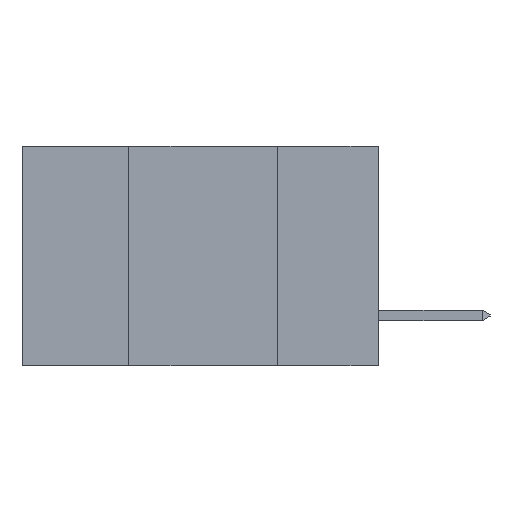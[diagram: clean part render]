
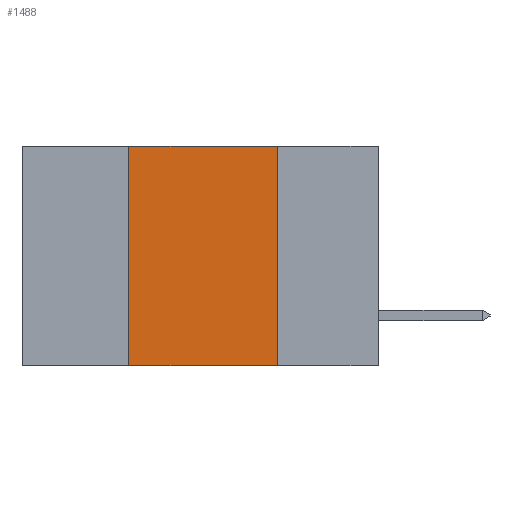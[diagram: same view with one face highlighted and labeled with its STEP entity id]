
A CAD part, left-side view. The second image highlights one B-rep face of the part: STEP entity #1488.
In plain terms, the highlighted planar face has unit normal (-1, 0, 0).
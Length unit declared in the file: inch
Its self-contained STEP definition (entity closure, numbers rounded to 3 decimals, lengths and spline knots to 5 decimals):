
#536 = EDGE_CURVE ( 'NONE', #11362, #21036, #21791, .T. ) ;
#632 = DIRECTION ( 'NONE',  ( 1., 0., 0. ) ) ;
#681 = LINE ( 'NONE', #11718, #6094 ) ;
#851 = CARTESIAN_POINT ( 'NONE',  ( 0., 0.17, -0.37 ) ) ;
#1311 = FACE_OUTER_BOUND ( 'NONE', #25648, .T. ) ;
#1488 = ADVANCED_FACE ( 'NONE', ( #1311 ), #12599, .F. ) ;
#1625 = EDGE_CURVE ( 'NONE', #11362, #15952, #23590, .T. ) ;
#1822 = CARTESIAN_POINT ( 'NONE',  ( 0., 0.6, 0. ) ) ;
#5709 = ORIENTED_EDGE ( 'NONE', *, *, #1625, .F. ) ;
#6094 = VECTOR ( 'NONE', #13730, 39.37008 ) ;
#8580 = LINE ( 'NONE', #1822, #13304 ) ;
#8680 = CARTESIAN_POINT ( 'NONE',  ( 0., 0.42, 0. ) ) ;
#10123 = ORIENTED_EDGE ( 'NONE', *, *, #10970, .F. ) ;
#10324 = ORIENTED_EDGE ( 'NONE', *, *, #12547, .F. ) ;
#10660 = VECTOR ( 'NONE', #20981, 39.37008 ) ;
#10970 = EDGE_CURVE ( 'NONE', #14653, #21036, #681, .T. ) ;
#11362 = VERTEX_POINT ( 'NONE', #15880 ) ;
#11718 = CARTESIAN_POINT ( 'NONE',  ( 0., 0.17, 0. ) ) ;
#11868 = CARTESIAN_POINT ( 'NONE',  ( 0., 0.6, 0. ) ) ;
#12547 = EDGE_CURVE ( 'NONE', #15952, #14653, #8580, .T. ) ;
#12599 = PLANE ( 'NONE',  #17858 ) ;
#13304 = VECTOR ( 'NONE', #19921, 39.37008 ) ;
#13730 = DIRECTION ( 'NONE',  ( 0., 0., -1. ) ) ;
#14105 = DIRECTION ( 'NONE',  ( 0., 0., 1. ) ) ;
#14653 = VERTEX_POINT ( 'NONE', #14657 ) ;
#14657 = CARTESIAN_POINT ( 'NONE',  ( 0., 0.17, 0. ) ) ;
#15880 = CARTESIAN_POINT ( 'NONE',  ( 0., 0.42, -0.37 ) ) ;
#15952 = VERTEX_POINT ( 'NONE', #8680 ) ;
#17292 = ORIENTED_EDGE ( 'NONE', *, *, #536, .T. ) ;
#17858 = AXIS2_PLACEMENT_3D ( 'NONE', #11868, #632, #22557 ) ;
#17954 = CARTESIAN_POINT ( 'NONE',  ( 0., 0.42, 0. ) ) ;
#18361 = VECTOR ( 'NONE', #14105, 39.37008 ) ;
#19921 = DIRECTION ( 'NONE',  ( 0., -1., 0. ) ) ;
#20421 = CARTESIAN_POINT ( 'NONE',  ( 0., 0.6, -0.37 ) ) ;
#20981 = DIRECTION ( 'NONE',  ( 0., -1., 0. ) ) ;
#21036 = VERTEX_POINT ( 'NONE', #851 ) ;
#21791 = LINE ( 'NONE', #20421, #10660 ) ;
#22557 = DIRECTION ( 'NONE',  ( 0., 0., -1. ) ) ;
#23590 = LINE ( 'NONE', #17954, #18361 ) ;
#25648 = EDGE_LOOP ( 'NONE', ( #10123, #10324, #5709, #17292 ) ) ;
